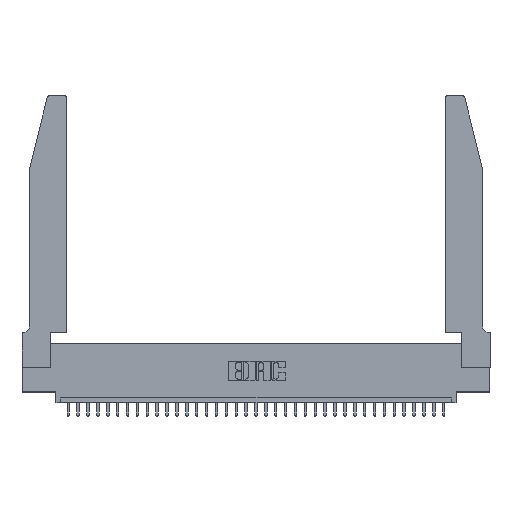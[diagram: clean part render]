
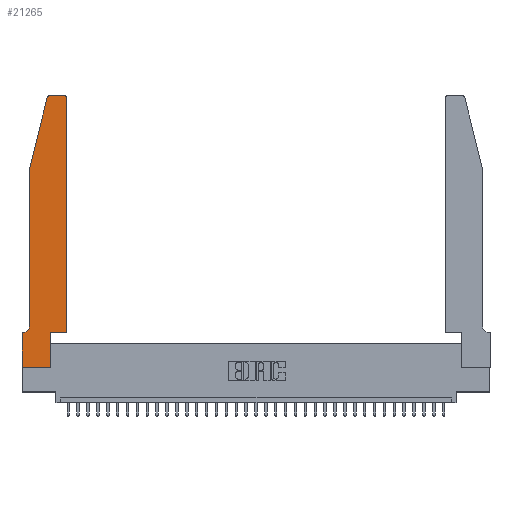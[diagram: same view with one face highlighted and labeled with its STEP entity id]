
A CAD part, top view. The second image highlights one B-rep face of the part: STEP entity #21265.
In plain terms, the highlighted planar face has unit normal (0, 0, 1).
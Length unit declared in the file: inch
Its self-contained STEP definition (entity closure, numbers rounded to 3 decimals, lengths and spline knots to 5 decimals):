
#1359 = ORIENTED_EDGE ( 'NONE', *, *, #11524, .T. ) ;
#2159 = VECTOR ( 'NONE', #11062, 39.37008 ) ;
#2302 = EDGE_CURVE ( 'NONE', #30047, #9500, #23679, .T. ) ;
#2560 = LINE ( 'NONE', #26696, #2159 ) ;
#3714 = EDGE_CURVE ( 'NONE', #14154, #20372, #24382, .T. ) ;
#4356 = AXIS2_PLACEMENT_3D ( 'NONE', #30383, #33072, #17079 ) ;
#4506 = ORIENTED_EDGE ( 'NONE', *, *, #22065, .T. ) ;
#4597 = CARTESIAN_POINT ( 'NONE',  ( 0.4505, 0.35, 0.37 ) ) ;
#4913 = EDGE_CURVE ( 'NONE', #14556, #8476, #19760, .T. ) ;
#5041 = DIRECTION ( 'NONE',  ( 1., 0., 0. ) ) ;
#5241 = ORIENTED_EDGE ( 'NONE', *, *, #14653, .T. ) ;
#5441 = VERTEX_POINT ( 'NONE', #21262 ) ;
#5691 = VERTEX_POINT ( 'NONE', #6622 ) ;
#5694 = AXIS2_PLACEMENT_3D ( 'NONE', #26773, #18157, #28999 ) ;
#5912 = CARTESIAN_POINT ( 'NONE',  ( 0.0055, 0.35, 0.37 ) ) ;
#6099 = DIRECTION ( 'NONE',  ( -0.239, -0.971, 0. ) ) ;
#6138 = CARTESIAN_POINT ( 'NONE',  ( 0.4505, 2.72, 0.37 ) ) ;
#6165 = CARTESIAN_POINT ( 'NONE',  ( 0.4505, 0.35, 0.37 ) ) ;
#6573 = CARTESIAN_POINT ( 'NONE',  ( 0.0755, 2., 0.37 ) ) ;
#6603 = LINE ( 'NONE', #18006, #11167 ) ;
#6622 = CARTESIAN_POINT ( 'NONE',  ( 0.2865, 0., 0.37 ) ) ;
#6767 = VECTOR ( 'NONE', #5041, 39.37008 ) ;
#7013 = CARTESIAN_POINT ( 'NONE',  ( 0.25487, 2.72718, 0.37 ) ) ;
#7232 = AXIS2_PLACEMENT_3D ( 'NONE', #32707, #13882, #32482 ) ;
#7481 = EDGE_CURVE ( 'NONE', #28139, #29714, #24706, .T. ) ;
#8309 = CARTESIAN_POINT ( 'NONE',  ( 0.0755, 2., 0.37 ) ) ;
#8476 = VERTEX_POINT ( 'NONE', #12478 ) ;
#8528 = CIRCLE ( 'NONE', #14523, 0.07 ) ;
#9339 = ORIENTED_EDGE ( 'NONE', *, *, #4913, .T. ) ;
#9500 = VERTEX_POINT ( 'NONE', #34083 ) ;
#9519 = VECTOR ( 'NONE', #11179, 39.37008 ) ;
#9593 = ORIENTED_EDGE ( 'NONE', *, *, #24970, .T. ) ;
#9616 = VECTOR ( 'NONE', #31107, 39.37008 ) ;
#9696 = VECTOR ( 'NONE', #20527, 39.37008 ) ;
#9746 = CARTESIAN_POINT ( 'NONE',  ( 0.0755, 0.35, 0.37 ) ) ;
#9802 = CARTESIAN_POINT ( 'NONE',  ( 0., 0., 0.37 ) ) ;
#10943 = ORIENTED_EDGE ( 'NONE', *, *, #21177, .T. ) ;
#11013 = DIRECTION ( 'NONE',  ( 0., -1., 0. ) ) ;
#11062 = DIRECTION ( 'NONE',  ( -1., 0., 0. ) ) ;
#11167 = VECTOR ( 'NONE', #19718, 39.37008 ) ;
#11179 = DIRECTION ( 'NONE',  ( 0., 1., 0. ) ) ;
#11484 = CARTESIAN_POINT ( 'NONE',  ( 0.0055, 0.42, 0.37 ) ) ;
#11524 = EDGE_CURVE ( 'NONE', #9500, #25257, #8528, .T. ) ;
#11577 = CARTESIAN_POINT ( 'NONE',  ( 0.0755, 2., 0.37 ) ) ;
#11835 = ORIENTED_EDGE ( 'NONE', *, *, #15605, .T. ) ;
#11996 = LINE ( 'NONE', #6165, #9519 ) ;
#12177 = LINE ( 'NONE', #31146, #9696 ) ;
#12478 = CARTESIAN_POINT ( 'NONE',  ( 0.4205, 2.75, 0.37 ) ) ;
#12875 = FACE_OUTER_BOUND ( 'NONE', #31487, .T. ) ;
#13882 = DIRECTION ( 'NONE',  ( 0., 0., 1. ) ) ;
#14154 = VERTEX_POINT ( 'NONE', #27373 ) ;
#14167 = LINE ( 'NONE', #9746, #9616 ) ;
#14312 = ORIENTED_EDGE ( 'NONE', *, *, #33760, .T. ) ;
#14523 = AXIS2_PLACEMENT_3D ( 'NONE', #11484, #19560, #19303 ) ;
#14556 = VERTEX_POINT ( 'NONE', #6138 ) ;
#14653 = EDGE_CURVE ( 'NONE', #25257, #5441, #14167, .T. ) ;
#15605 = EDGE_CURVE ( 'NONE', #5691, #28139, #6603, .T. ) ;
#16573 = CARTESIAN_POINT ( 'NONE',  ( 0.2865, 0.35, 0.37 ) ) ;
#17079 = DIRECTION ( 'NONE',  ( 1., 0., 0. ) ) ;
#18006 = CARTESIAN_POINT ( 'NONE',  ( 0.2865, 0.35, 0.37 ) ) ;
#18157 = DIRECTION ( 'NONE',  ( 0., 0., 1. ) ) ;
#19137 = VECTOR ( 'NONE', #6099, 39.37008 ) ;
#19303 = DIRECTION ( 'NONE',  ( -1., 0., 0. ) ) ;
#19460 = VECTOR ( 'NONE', #32450, 39.37008 ) ;
#19560 = DIRECTION ( 'NONE',  ( 0., 0., -1. ) ) ;
#19718 = DIRECTION ( 'NONE',  ( 0., 1., 0. ) ) ;
#19760 = CIRCLE ( 'NONE', #5694, 0.03 ) ;
#20004 = LINE ( 'NONE', #6573, #19137 ) ;
#20372 = VERTEX_POINT ( 'NONE', #7013 ) ;
#20419 = ORIENTED_EDGE ( 'NONE', *, *, #2302, .T. ) ;
#20527 = DIRECTION ( 'NONE',  ( 1., 0., 0. ) ) ;
#21177 = EDGE_CURVE ( 'NONE', #20372, #30047, #20004, .T. ) ;
#21262 = CARTESIAN_POINT ( 'NONE',  ( 0., 0.35, 0.37 ) ) ;
#21265 = ADVANCED_FACE ( 'NONE', ( #12875 ), #27671, .T. ) ;
#22065 = EDGE_CURVE ( 'NONE', #5441, #28906, #28249, .T. ) ;
#23679 = LINE ( 'NONE', #8309, #19460 ) ;
#24382 = CIRCLE ( 'NONE', #7232, 0.03 ) ;
#24627 = EDGE_CURVE ( 'NONE', #28906, #5691, #12177, .T. ) ;
#24706 = LINE ( 'NONE', #27889, #6767 ) ;
#24970 = EDGE_CURVE ( 'NONE', #29714, #14556, #11996, .T. ) ;
#25257 = VERTEX_POINT ( 'NONE', #5912 ) ;
#26696 = CARTESIAN_POINT ( 'NONE',  ( 0.2605, 2.75, 0.37 ) ) ;
#26773 = CARTESIAN_POINT ( 'NONE',  ( 0.4205, 2.72, 0.37 ) ) ;
#27373 = CARTESIAN_POINT ( 'NONE',  ( 0.284, 2.75, 0.37 ) ) ;
#27410 = ORIENTED_EDGE ( 'NONE', *, *, #7481, .T. ) ;
#27671 = PLANE ( 'NONE',  #4356 ) ;
#27889 = CARTESIAN_POINT ( 'NONE',  ( 0.4505, 0.35, 0.37 ) ) ;
#28131 = ORIENTED_EDGE ( 'NONE', *, *, #3714, .T. ) ;
#28139 = VERTEX_POINT ( 'NONE', #16573 ) ;
#28249 = LINE ( 'NONE', #29244, #30371 ) ;
#28906 = VERTEX_POINT ( 'NONE', #9802 ) ;
#28999 = DIRECTION ( 'NONE',  ( 1., 0., 0. ) ) ;
#29244 = CARTESIAN_POINT ( 'NONE',  ( 0., 0., 0.37 ) ) ;
#29586 = ORIENTED_EDGE ( 'NONE', *, *, #24627, .T. ) ;
#29714 = VERTEX_POINT ( 'NONE', #4597 ) ;
#30047 = VERTEX_POINT ( 'NONE', #11577 ) ;
#30371 = VECTOR ( 'NONE', #11013, 39.37008 ) ;
#30383 = CARTESIAN_POINT ( 'NONE',  ( 0., 0.35, 0.37 ) ) ;
#31107 = DIRECTION ( 'NONE',  ( -1., 0., 0. ) ) ;
#31146 = CARTESIAN_POINT ( 'NONE',  ( 0., 0., 0.37 ) ) ;
#31487 = EDGE_LOOP ( 'NONE', ( #14312, #28131, #10943, #20419, #1359, #5241, #4506, #29586, #11835, #27410, #9593, #9339 ) ) ;
#32450 = DIRECTION ( 'NONE',  ( 0., -1., 0. ) ) ;
#32482 = DIRECTION ( 'NONE',  ( 1., 0., 0. ) ) ;
#32707 = CARTESIAN_POINT ( 'NONE',  ( 0.284, 2.72, 0.37 ) ) ;
#33072 = DIRECTION ( 'NONE',  ( 0., 0., 1. ) ) ;
#33760 = EDGE_CURVE ( 'NONE', #8476, #14154, #2560, .T. ) ;
#34083 = CARTESIAN_POINT ( 'NONE',  ( 0.0755, 0.42, 0.37 ) ) ;
